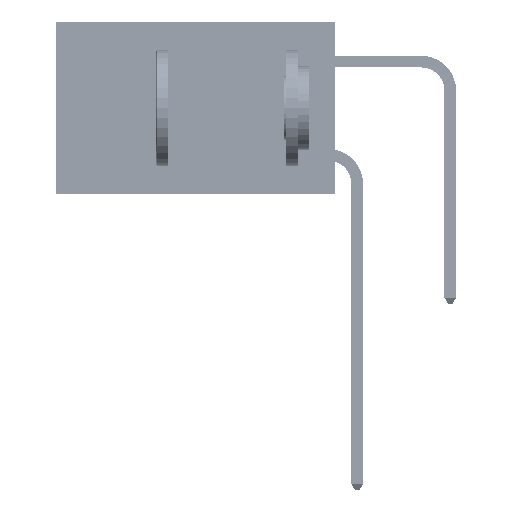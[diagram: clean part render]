
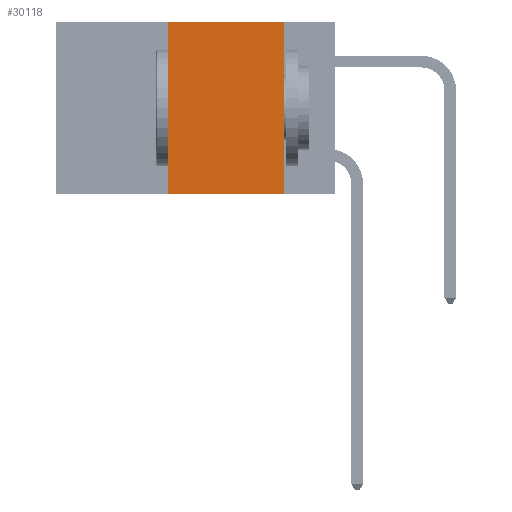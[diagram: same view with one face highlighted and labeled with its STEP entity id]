
A CAD part, left-side view. The second image highlights one B-rep face of the part: STEP entity #30118.
In plain terms, the highlighted planar face has unit normal (-1, 0, 0).
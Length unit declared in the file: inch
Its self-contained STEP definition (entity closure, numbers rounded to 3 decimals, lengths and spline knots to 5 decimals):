
#1616 = DIRECTION ( 'NONE',  ( 0., -1., 0. ) ) ;
#8816 = VECTOR ( 'NONE', #27189, 39.37008 ) ;
#10797 = ORIENTED_EDGE ( 'NONE', *, *, #47679, .F. ) ;
#11590 = EDGE_CURVE ( 'NONE', #42550, #15182, #50622, .T. ) ;
#15182 = VERTEX_POINT ( 'NONE', #23869 ) ;
#16395 = VECTOR ( 'NONE', #52788, 39.37008 ) ;
#16535 = DIRECTION ( 'NONE',  ( 0., 0., -1. ) ) ;
#16714 = PLANE ( 'NONE',  #40766 ) ;
#22085 = EDGE_CURVE ( 'NONE', #46617, #39060, #36765, .T. ) ;
#22727 = CARTESIAN_POINT ( 'NONE',  ( 0., 0.36, 0. ) ) ;
#23815 = DIRECTION ( 'NONE',  ( 0., 0., -1. ) ) ;
#23869 = CARTESIAN_POINT ( 'NONE',  ( 0., 0.11, -0.37 ) ) ;
#27098 = CARTESIAN_POINT ( 'NONE',  ( 0., 0.6, -0.37 ) ) ;
#27189 = DIRECTION ( 'NONE',  ( 0., 0., 1. ) ) ;
#28250 = CARTESIAN_POINT ( 'NONE',  ( 0., 0.36, 0. ) ) ;
#30118 = ADVANCED_FACE ( 'NONE', ( #49416 ), #16714, .F. ) ;
#30694 = CARTESIAN_POINT ( 'NONE',  ( 0., 0.36, -0.37 ) ) ;
#32886 = VECTOR ( 'NONE', #1616, 39.37008 ) ;
#33590 = ORIENTED_EDGE ( 'NONE', *, *, #11590, .F. ) ;
#36765 = LINE ( 'NONE', #22727, #8816 ) ;
#37939 = ORIENTED_EDGE ( 'NONE', *, *, #39569, .T. ) ;
#39060 = VERTEX_POINT ( 'NONE', #28250 ) ;
#39569 = EDGE_CURVE ( 'NONE', #46617, #15182, #54737, .T. ) ;
#40766 = AXIS2_PLACEMENT_3D ( 'NONE', #46511, #46344, #16535 ) ;
#42550 = VERTEX_POINT ( 'NONE', #45075 ) ;
#42700 = VECTOR ( 'NONE', #23815, 39.37008 ) ;
#45075 = CARTESIAN_POINT ( 'NONE',  ( 0., 0.11, 0. ) ) ;
#46344 = DIRECTION ( 'NONE',  ( 1., 0., 0. ) ) ;
#46511 = CARTESIAN_POINT ( 'NONE',  ( 0., 0.6, 0. ) ) ;
#46617 = VERTEX_POINT ( 'NONE', #30694 ) ;
#47679 = EDGE_CURVE ( 'NONE', #39060, #42550, #49552, .T. ) ;
#47991 = CARTESIAN_POINT ( 'NONE',  ( 0., 0.6, 0. ) ) ;
#49416 = FACE_OUTER_BOUND ( 'NONE', #54587, .T. ) ;
#49552 = LINE ( 'NONE', #47991, #16395 ) ;
#50622 = LINE ( 'NONE', #53792, #42700 ) ;
#51856 = ORIENTED_EDGE ( 'NONE', *, *, #22085, .F. ) ;
#52788 = DIRECTION ( 'NONE',  ( 0., -1., 0. ) ) ;
#53792 = CARTESIAN_POINT ( 'NONE',  ( 0., 0.11, 0. ) ) ;
#54587 = EDGE_LOOP ( 'NONE', ( #33590, #10797, #51856, #37939 ) ) ;
#54737 = LINE ( 'NONE', #27098, #32886 ) ;
